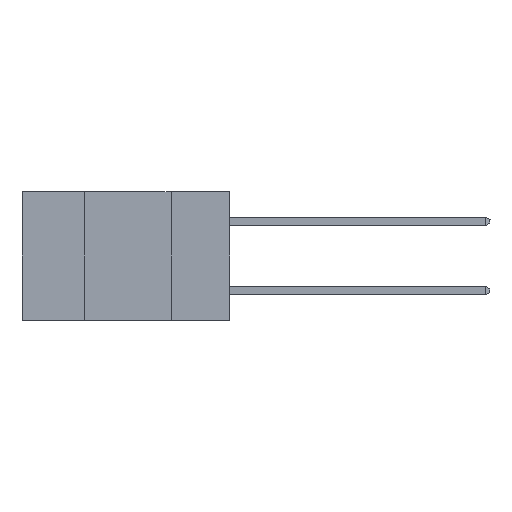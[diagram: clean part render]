
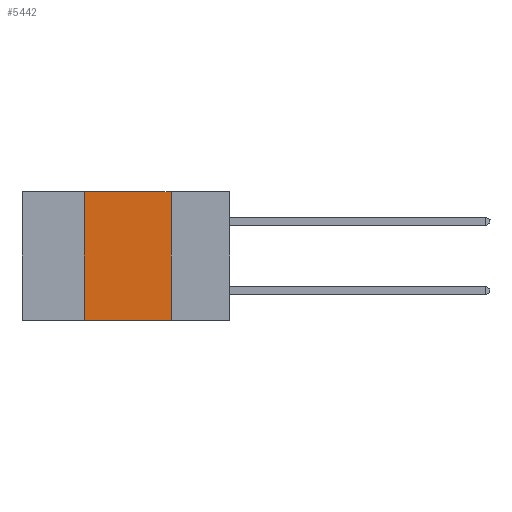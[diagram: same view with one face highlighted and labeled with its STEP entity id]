
A CAD part, left-side view. The second image highlights one B-rep face of the part: STEP entity #5442.
In plain terms, the highlighted planar face has unit normal (-1, 0, 0).
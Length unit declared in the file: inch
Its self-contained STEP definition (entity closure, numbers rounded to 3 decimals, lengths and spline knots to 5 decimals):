
#816 = FACE_OUTER_BOUND ( 'NONE', #10216, .T. ) ;
#1895 = VECTOR ( 'NONE', #5439, 39.37008 ) ;
#2157 = CARTESIAN_POINT ( 'NONE',  ( 0., 0.17, 0. ) ) ;
#2219 = AXIS2_PLACEMENT_3D ( 'NONE', #16168, #10253, #3034 ) ;
#2238 = CARTESIAN_POINT ( 'NONE',  ( 0., 0.17, -0.37 ) ) ;
#2708 = DIRECTION ( 'NONE',  ( 0., 0., -1. ) ) ;
#2928 = LINE ( 'NONE', #17388, #14788 ) ;
#3034 = DIRECTION ( 'NONE',  ( 0., 0., -1. ) ) ;
#3095 = PLANE ( 'NONE',  #2219 ) ;
#3112 = VERTEX_POINT ( 'NONE', #2157 ) ;
#3117 = CARTESIAN_POINT ( 'NONE',  ( 0., 0.42, -0.37 ) ) ;
#3458 = LINE ( 'NONE', #5166, #15559 ) ;
#3529 = VERTEX_POINT ( 'NONE', #3117 ) ;
#4015 = CARTESIAN_POINT ( 'NONE',  ( 0., 0.17, 0. ) ) ;
#5166 = CARTESIAN_POINT ( 'NONE',  ( 0., 0.42, 0. ) ) ;
#5265 = CARTESIAN_POINT ( 'NONE',  ( 0., 0.42, 0. ) ) ;
#5439 = DIRECTION ( 'NONE',  ( 0., -1., 0. ) ) ;
#5442 = ADVANCED_FACE ( 'NONE', ( #816 ), #3095, .F. ) ;
#7195 = ORIENTED_EDGE ( 'NONE', *, *, #8662, .F. ) ;
#8662 = EDGE_CURVE ( 'NONE', #3112, #8724, #12553, .T. ) ;
#8724 = VERTEX_POINT ( 'NONE', #2238 ) ;
#9385 = ORIENTED_EDGE ( 'NONE', *, *, #15772, .F. ) ;
#9546 = VERTEX_POINT ( 'NONE', #5265 ) ;
#9560 = ORIENTED_EDGE ( 'NONE', *, *, #11431, .T. ) ;
#10216 = EDGE_LOOP ( 'NONE', ( #7195, #12865, #9385, #9560 ) ) ;
#10253 = DIRECTION ( 'NONE',  ( 1., 0., 0. ) ) ;
#11431 = EDGE_CURVE ( 'NONE', #3529, #8724, #16212, .T. ) ;
#11649 = VECTOR ( 'NONE', #2708, 39.37008 ) ;
#12553 = LINE ( 'NONE', #4015, #11649 ) ;
#12865 = ORIENTED_EDGE ( 'NONE', *, *, #14305, .F. ) ;
#13246 = DIRECTION ( 'NONE',  ( 0., -1., 0. ) ) ;
#14305 = EDGE_CURVE ( 'NONE', #9546, #3112, #2928, .T. ) ;
#14788 = VECTOR ( 'NONE', #13246, 39.37008 ) ;
#15559 = VECTOR ( 'NONE', #15577, 39.37008 ) ;
#15577 = DIRECTION ( 'NONE',  ( 0., 0., 1. ) ) ;
#15697 = CARTESIAN_POINT ( 'NONE',  ( 0., 0.6, -0.37 ) ) ;
#15772 = EDGE_CURVE ( 'NONE', #3529, #9546, #3458, .T. ) ;
#16168 = CARTESIAN_POINT ( 'NONE',  ( 0., 0.6, 0. ) ) ;
#16212 = LINE ( 'NONE', #15697, #1895 ) ;
#17388 = CARTESIAN_POINT ( 'NONE',  ( 0., 0.6, 0. ) ) ;
